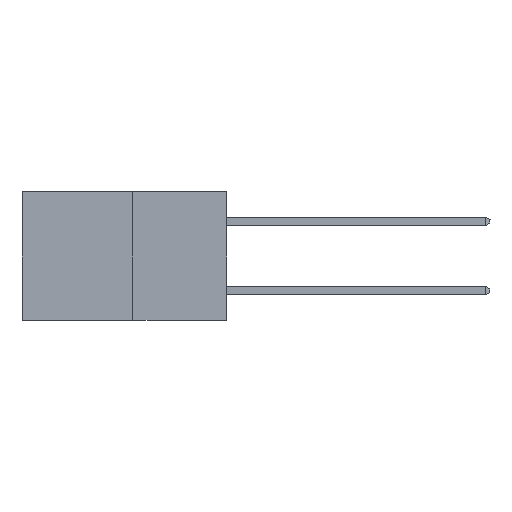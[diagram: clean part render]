
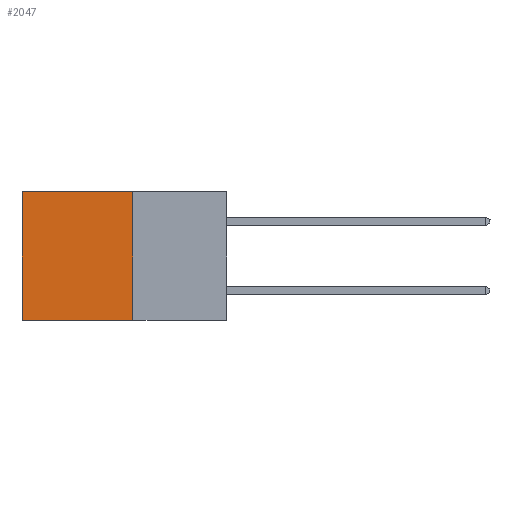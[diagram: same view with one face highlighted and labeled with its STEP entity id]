
A CAD part, left-side view. The second image highlights one B-rep face of the part: STEP entity #2047.
In plain terms, the highlighted planar face has unit normal (-1, 0, 0).
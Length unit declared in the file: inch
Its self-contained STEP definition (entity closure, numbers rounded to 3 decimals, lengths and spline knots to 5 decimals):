
#133 = CARTESIAN_POINT ( 'NONE',  ( 0.277, 0.27, 0. ) ) ;
#1550 = LINE ( 'NONE', #16739, #15564 ) ;
#1876 = VERTEX_POINT ( 'NONE', #6623 ) ;
#1969 = VECTOR ( 'NONE', #4358, 39.37008 ) ;
#2047 = ADVANCED_FACE ( 'NONE', ( #16752 ), #16177, .F. ) ;
#3104 = ORIENTED_EDGE ( 'NONE', *, *, #9647, .T. ) ;
#4238 = ORIENTED_EDGE ( 'NONE', *, *, #7802, .F. ) ;
#4358 = DIRECTION ( 'NONE',  ( 0., 0., -1. ) ) ;
#4363 = ORIENTED_EDGE ( 'NONE', *, *, #12089, .F. ) ;
#5164 = EDGE_CURVE ( 'NONE', #15572, #9062, #11673, .T. ) ;
#5979 = CARTESIAN_POINT ( 'NONE',  ( 0.277, 0.59, -0.37 ) ) ;
#6623 = CARTESIAN_POINT ( 'NONE',  ( 0.277, 0.27, -0.37 ) ) ;
#7802 = EDGE_CURVE ( 'NONE', #9043, #1876, #17176, .T. ) ;
#7824 = CARTESIAN_POINT ( 'NONE',  ( 0.277, 0.59, 0. ) ) ;
#7936 = EDGE_LOOP ( 'NONE', ( #23779, #4363, #4238, #3104 ) ) ;
#9043 = VERTEX_POINT ( 'NONE', #133 ) ;
#9062 = VERTEX_POINT ( 'NONE', #5979 ) ;
#9647 = EDGE_CURVE ( 'NONE', #9043, #15572, #20422, .T. ) ;
#11104 = DIRECTION ( 'NONE',  ( 0., 1., 0. ) ) ;
#11263 = CARTESIAN_POINT ( 'NONE',  ( 0.277, 0.27, -0.37 ) ) ;
#11673 = LINE ( 'NONE', #23468, #16708 ) ;
#12089 = EDGE_CURVE ( 'NONE', #1876, #9062, #1550, .T. ) ;
#12365 = DIRECTION ( 'NONE',  ( 1., 0., 0. ) ) ;
#13215 = CARTESIAN_POINT ( 'NONE',  ( 0.277, 0.27, 0. ) ) ;
#13465 = DIRECTION ( 'NONE',  ( 0., 0., -1. ) ) ;
#15385 = VECTOR ( 'NONE', #17044, 39.37008 ) ;
#15564 = VECTOR ( 'NONE', #11104, 39.37008 ) ;
#15572 = VERTEX_POINT ( 'NONE', #7824 ) ;
#16177 = PLANE ( 'NONE',  #21483 ) ;
#16708 = VECTOR ( 'NONE', #23340, 39.37008 ) ;
#16739 = CARTESIAN_POINT ( 'NONE',  ( 0.277, 0.27, -0.37 ) ) ;
#16752 = FACE_OUTER_BOUND ( 'NONE', #7936, .T. ) ;
#17044 = DIRECTION ( 'NONE',  ( 0., 1., 0. ) ) ;
#17176 = LINE ( 'NONE', #23153, #1969 ) ;
#20422 = LINE ( 'NONE', #13215, #15385 ) ;
#21483 = AXIS2_PLACEMENT_3D ( 'NONE', #11263, #12365, #13465 ) ;
#23153 = CARTESIAN_POINT ( 'NONE',  ( 0.277, 0.27, -0.37 ) ) ;
#23340 = DIRECTION ( 'NONE',  ( 0., 0., -1. ) ) ;
#23468 = CARTESIAN_POINT ( 'NONE',  ( 0.277, 0.59, -0.37 ) ) ;
#23779 = ORIENTED_EDGE ( 'NONE', *, *, #5164, .T. ) ;
